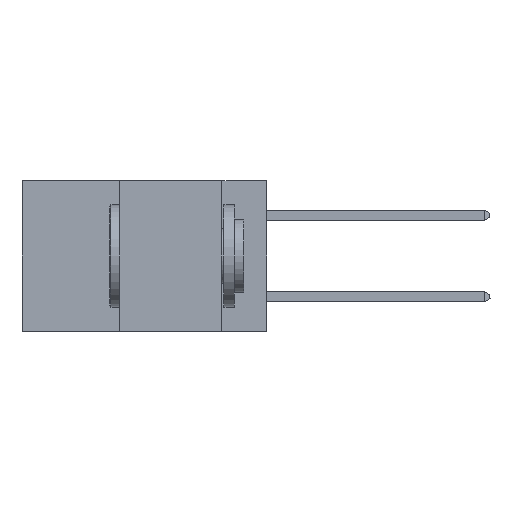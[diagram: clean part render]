
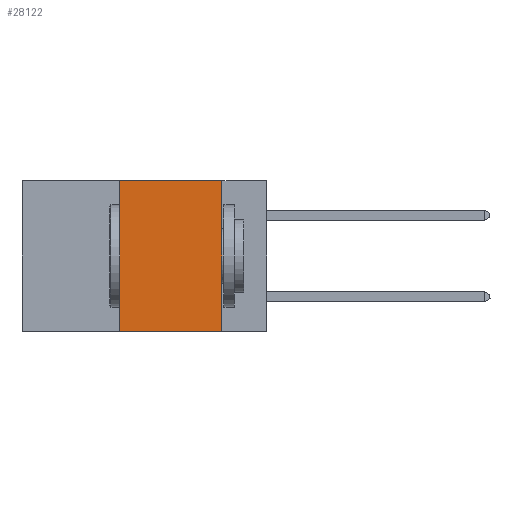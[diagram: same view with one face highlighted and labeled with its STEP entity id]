
A CAD part, left-side view. The second image highlights one B-rep face of the part: STEP entity #28122.
In plain terms, the highlighted planar face has unit normal (-1, 0, 0).
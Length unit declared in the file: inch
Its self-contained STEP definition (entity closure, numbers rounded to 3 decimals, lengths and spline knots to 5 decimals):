
#662 = LINE ( 'NONE', #23848, #21106 ) ;
#695 = VECTOR ( 'NONE', #12314, 39.37008 ) ;
#1226 = CARTESIAN_POINT ( 'NONE',  ( 0., 0.36, 0. ) ) ;
#1427 = CARTESIAN_POINT ( 'NONE',  ( 0., 0.11, -0.37 ) ) ;
#2144 = EDGE_LOOP ( 'NONE', ( #33349, #4920, #18429, #5935 ) ) ;
#2306 = CARTESIAN_POINT ( 'NONE',  ( 0., 0.6, -0.37 ) ) ;
#2575 = VERTEX_POINT ( 'NONE', #28013 ) ;
#2972 = FACE_OUTER_BOUND ( 'NONE', #2144, .T. ) ;
#3605 = DIRECTION ( 'NONE',  ( 0., 0., 1. ) ) ;
#3850 = AXIS2_PLACEMENT_3D ( 'NONE', #20761, #17690, #17912 ) ;
#4920 = ORIENTED_EDGE ( 'NONE', *, *, #5130, .F. ) ;
#5130 = EDGE_CURVE ( 'NONE', #14019, #2575, #31083, .T. ) ;
#5935 = ORIENTED_EDGE ( 'NONE', *, *, #11479, .T. ) ;
#5992 = CARTESIAN_POINT ( 'NONE',  ( 0., 0.36, 0. ) ) ;
#9756 = VECTOR ( 'NONE', #3605, 39.37008 ) ;
#9924 = CARTESIAN_POINT ( 'NONE',  ( 0., 0.36, -0.37 ) ) ;
#10350 = CARTESIAN_POINT ( 'NONE',  ( 0., 0.6, 0. ) ) ;
#11479 = EDGE_CURVE ( 'NONE', #24572, #33220, #12921, .T. ) ;
#11748 = LINE ( 'NONE', #5992, #9756 ) ;
#11775 = EDGE_CURVE ( 'NONE', #2575, #33220, #662, .T. ) ;
#12314 = DIRECTION ( 'NONE',  ( 0., -1., 0. ) ) ;
#12921 = LINE ( 'NONE', #2306, #695 ) ;
#14019 = VERTEX_POINT ( 'NONE', #1226 ) ;
#17690 = DIRECTION ( 'NONE',  ( 1., 0., 0. ) ) ;
#17912 = DIRECTION ( 'NONE',  ( 0., 0., -1. ) ) ;
#18429 = ORIENTED_EDGE ( 'NONE', *, *, #31147, .F. ) ;
#20493 = VECTOR ( 'NONE', #23493, 39.37008 ) ;
#20761 = CARTESIAN_POINT ( 'NONE',  ( 0., 0.6, 0. ) ) ;
#21106 = VECTOR ( 'NONE', #23616, 39.37008 ) ;
#23493 = DIRECTION ( 'NONE',  ( 0., -1., 0. ) ) ;
#23616 = DIRECTION ( 'NONE',  ( 0., 0., -1. ) ) ;
#23848 = CARTESIAN_POINT ( 'NONE',  ( 0., 0.11, 0. ) ) ;
#24572 = VERTEX_POINT ( 'NONE', #9924 ) ;
#26013 = PLANE ( 'NONE',  #3850 ) ;
#28013 = CARTESIAN_POINT ( 'NONE',  ( 0., 0.11, 0. ) ) ;
#28122 = ADVANCED_FACE ( 'NONE', ( #2972 ), #26013, .F. ) ;
#31083 = LINE ( 'NONE', #10350, #20493 ) ;
#31147 = EDGE_CURVE ( 'NONE', #24572, #14019, #11748, .T. ) ;
#33220 = VERTEX_POINT ( 'NONE', #1427 ) ;
#33349 = ORIENTED_EDGE ( 'NONE', *, *, #11775, .F. ) ;
